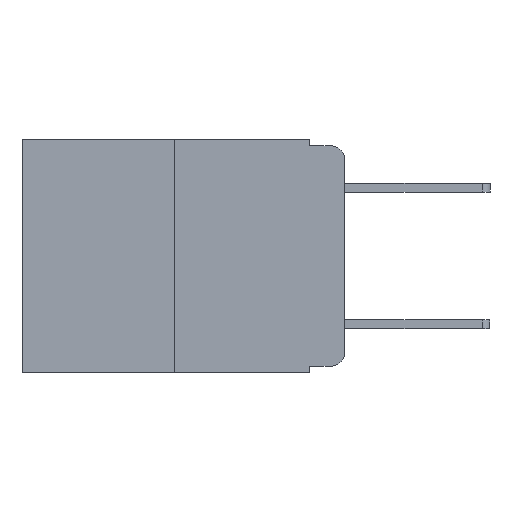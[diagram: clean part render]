
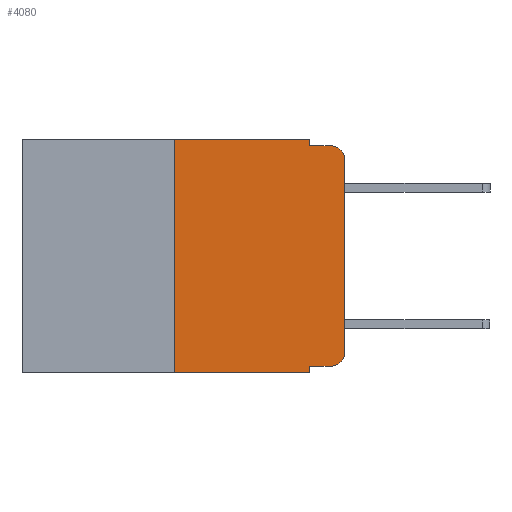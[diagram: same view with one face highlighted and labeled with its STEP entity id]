
A CAD part, left-side view. The second image highlights one B-rep face of the part: STEP entity #4080.
In plain terms, the highlighted planar face has unit normal (-1, 0, 0).
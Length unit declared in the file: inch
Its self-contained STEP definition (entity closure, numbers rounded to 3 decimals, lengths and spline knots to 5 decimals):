
#67 = LINE ( 'NONE', #9788, #9974 ) ;
#305 = CARTESIAN_POINT ( 'NONE',  ( 0., 0.25, 0. ) ) ;
#331 = ORIENTED_EDGE ( 'NONE', *, *, #6136, .F. ) ;
#448 = VECTOR ( 'NONE', #3157, 39.37008 ) ;
#677 = VERTEX_POINT ( 'NONE', #6390 ) ;
#843 = EDGE_CURVE ( 'NONE', #11768, #5896, #10769, .T. ) ;
#1000 = VECTOR ( 'NONE', #6308, 39.37008 ) ;
#1386 = ORIENTED_EDGE ( 'NONE', *, *, #7308, .F. ) ;
#1390 = DIRECTION ( 'NONE',  ( 0., 0., 1. ) ) ;
#1550 = CARTESIAN_POINT ( 'NONE',  ( 0., 0.473, -0.343 ) ) ;
#1609 = VECTOR ( 'NONE', #2062, 39.37008 ) ;
#1746 = ORIENTED_EDGE ( 'NONE', *, *, #10855, .T. ) ;
#1916 = ORIENTED_EDGE ( 'NONE', *, *, #8957, .T. ) ;
#2062 = DIRECTION ( 'NONE',  ( 0., -1., 0. ) ) ;
#2098 = ORIENTED_EDGE ( 'NONE', *, *, #4319, .F. ) ;
#2157 = CARTESIAN_POINT ( 'NONE',  ( 0., 0.473, 0. ) ) ;
#2371 = VECTOR ( 'NONE', #9227, 39.37008 ) ;
#2428 = VERTEX_POINT ( 'NONE', #7215 ) ;
#2439 = CARTESIAN_POINT ( 'NONE',  ( 0., 0.02, -0.313 ) ) ;
#2581 = CIRCLE ( 'NONE', #11618, 0.02 ) ;
#2729 = DIRECTION ( 'NONE',  ( 1., 0., 0. ) ) ;
#3157 = DIRECTION ( 'NONE',  ( 0., -1., 0. ) ) ;
#3208 = LINE ( 'NONE', #2157, #448 ) ;
#3292 = ORIENTED_EDGE ( 'NONE', *, *, #4260, .F. ) ;
#3454 = DIRECTION ( 'NONE',  ( 0., 0., -1. ) ) ;
#3504 = FACE_OUTER_BOUND ( 'NONE', #8501, .T. ) ;
#3702 = CARTESIAN_POINT ( 'NONE',  ( 0., 0.051, 0. ) ) ;
#3759 = LINE ( 'NONE', #305, #7839 ) ;
#4080 = ADVANCED_FACE ( 'NONE', ( #3504 ), #4712, .F. ) ;
#4118 = CARTESIAN_POINT ( 'NONE',  ( 0., 0., -0.03 ) ) ;
#4260 = EDGE_CURVE ( 'NONE', #2428, #677, #10976, .T. ) ;
#4319 = EDGE_CURVE ( 'NONE', #7208, #5853, #3208, .T. ) ;
#4544 = ORIENTED_EDGE ( 'NONE', *, *, #8342, .F. ) ;
#4599 = DIRECTION ( 'NONE',  ( -1., 0., 0. ) ) ;
#4712 = PLANE ( 'NONE',  #4874 ) ;
#4874 = AXIS2_PLACEMENT_3D ( 'NONE', #9255, #2729, #5652 ) ;
#5262 = CARTESIAN_POINT ( 'NONE',  ( 0., 0.051, 0. ) ) ;
#5544 = DIRECTION ( 'NONE',  ( 0., -1., 0. ) ) ;
#5605 = ORIENTED_EDGE ( 'NONE', *, *, #5859, .T. ) ;
#5652 = DIRECTION ( 'NONE',  ( 0., 0., -1. ) ) ;
#5838 = CARTESIAN_POINT ( 'NONE',  ( 0., 0.051, -0.333 ) ) ;
#5853 = VERTEX_POINT ( 'NONE', #5262 ) ;
#5859 = EDGE_CURVE ( 'NONE', #7533, #7092, #67, .T. ) ;
#5873 = VERTEX_POINT ( 'NONE', #8008 ) ;
#5896 = VERTEX_POINT ( 'NONE', #11651 ) ;
#6037 = CARTESIAN_POINT ( 'NONE',  ( 0., 0.25, -0.343 ) ) ;
#6070 = EDGE_CURVE ( 'NONE', #7092, #677, #10406, .T. ) ;
#6136 = EDGE_CURVE ( 'NONE', #5853, #2428, #12243, .T. ) ;
#6182 = DIRECTION ( 'NONE',  ( 0., 0., 1. ) ) ;
#6308 = DIRECTION ( 'NONE',  ( 0., -1., 0. ) ) ;
#6390 = CARTESIAN_POINT ( 'NONE',  ( 0., 0.02, -0.01 ) ) ;
#6586 = CARTESIAN_POINT ( 'NONE',  ( 0., 0.051, 0. ) ) ;
#7092 = VERTEX_POINT ( 'NONE', #4118 ) ;
#7208 = VERTEX_POINT ( 'NONE', #8865 ) ;
#7215 = CARTESIAN_POINT ( 'NONE',  ( 0., 0.051, -0.01 ) ) ;
#7308 = EDGE_CURVE ( 'NONE', #11768, #7208, #3759, .T. ) ;
#7533 = VERTEX_POINT ( 'NONE', #9219 ) ;
#7535 = VECTOR ( 'NONE', #10189, 39.37008 ) ;
#7753 = VERTEX_POINT ( 'NONE', #5838 ) ;
#7839 = VECTOR ( 'NONE', #1390, 39.37008 ) ;
#8008 = CARTESIAN_POINT ( 'NONE',  ( 0., 0.02, -0.333 ) ) ;
#8265 = AXIS2_PLACEMENT_3D ( 'NONE', #10058, #4599, #10961 ) ;
#8342 = EDGE_CURVE ( 'NONE', #7753, #5896, #10208, .T. ) ;
#8501 = EDGE_LOOP ( 'NONE', ( #5605, #9910, #3292, #331, #2098, #1386, #11029, #4544, #1916, #1746 ) ) ;
#8675 = CARTESIAN_POINT ( 'NONE',  ( 0., 0.051, -0.01 ) ) ;
#8774 = VECTOR ( 'NONE', #5544, 39.37008 ) ;
#8865 = CARTESIAN_POINT ( 'NONE',  ( 0., 0.25, 0. ) ) ;
#8957 = EDGE_CURVE ( 'NONE', #7753, #5873, #10898, .T. ) ;
#9004 = DIRECTION ( 'NONE',  ( -1., 0., 0. ) ) ;
#9219 = CARTESIAN_POINT ( 'NONE',  ( 0., 0., -0.313 ) ) ;
#9227 = DIRECTION ( 'NONE',  ( 0., 0., -1. ) ) ;
#9255 = CARTESIAN_POINT ( 'NONE',  ( 0., 0.473, 0. ) ) ;
#9788 = CARTESIAN_POINT ( 'NONE',  ( 0., 0., 0. ) ) ;
#9910 = ORIENTED_EDGE ( 'NONE', *, *, #6070, .T. ) ;
#9974 = VECTOR ( 'NONE', #6182, 39.37008 ) ;
#10058 = CARTESIAN_POINT ( 'NONE',  ( 0., 0.02, -0.03 ) ) ;
#10059 = CARTESIAN_POINT ( 'NONE',  ( 0., 0.051, -0.333 ) ) ;
#10189 = DIRECTION ( 'NONE',  ( 0., 0., -1. ) ) ;
#10208 = LINE ( 'NONE', #6586, #7535 ) ;
#10406 = CIRCLE ( 'NONE', #8265, 0.02 ) ;
#10769 = LINE ( 'NONE', #1550, #1000 ) ;
#10855 = EDGE_CURVE ( 'NONE', #5873, #7533, #2581, .T. ) ;
#10898 = LINE ( 'NONE', #10059, #8774 ) ;
#10961 = DIRECTION ( 'NONE',  ( 0., 0., -1. ) ) ;
#10976 = LINE ( 'NONE', #8675, #1609 ) ;
#11029 = ORIENTED_EDGE ( 'NONE', *, *, #843, .T. ) ;
#11618 = AXIS2_PLACEMENT_3D ( 'NONE', #2439, #9004, #3454 ) ;
#11651 = CARTESIAN_POINT ( 'NONE',  ( 0., 0.051, -0.343 ) ) ;
#11768 = VERTEX_POINT ( 'NONE', #6037 ) ;
#12243 = LINE ( 'NONE', #3702, #2371 ) ;
